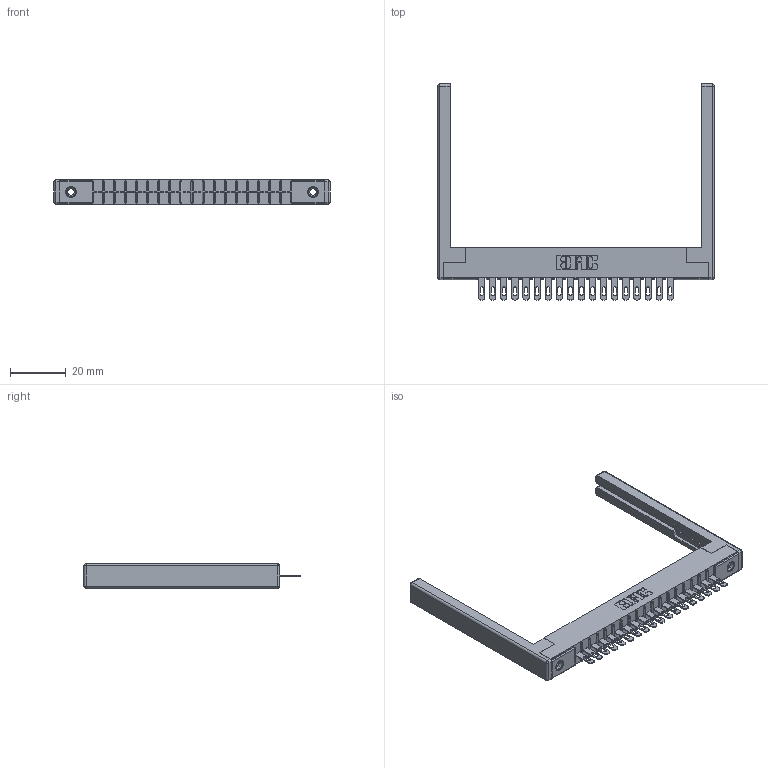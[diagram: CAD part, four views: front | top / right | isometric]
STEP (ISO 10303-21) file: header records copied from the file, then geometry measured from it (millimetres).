
FILE_DESCRIPTION (( 'STEP AP203' ), '1' );
FILE_NAME ('356-018-400-168.STEP', '2020-09-23T13:24:30', ( '' ), ( '' ), 'SwSTEP 2.0', 'SolidWorks 2020', '' );
FILE_SCHEMA (( 'CONFIG_CONTROL_DESIGN' ));
Length unit declared in the file: inch
Products named in the file (5): 306 Part_.156 Dia; 345-250-001_345-250-001-102; 356-018-400-168; 306-290-001_100; 307-220-068
Assembly tree (23 placements, depth 2):
  356-018-400-168
    306 Part_.156 Dia
    306-290-001_100  x18
    345-250-001_345-250-001-102  x2
    307-220-068  x2
Bounding box: 98.76 x 77.17 x 8.71 mm (x, y, z)
Volume: 11338.6 mm3; surface area: 14321.8 mm2
Topology: 23 solids, 23 shells, 1638 faces, 4576 edges, 2932 vertices
Faces by surface type: plane 1056, cylinder 486, sphere 80, cone 12, torus 4
Entity records: 22818 total; most frequent: CARTESIAN_POINT 3794, DIRECTION 3757, ORIENTED_EDGE 3750, EDGE_CURVE 1875, VECTOR 1447, LINE 1447, VERTEX_POINT 1192, AXIS2_PLACEMENT_3D 1155
